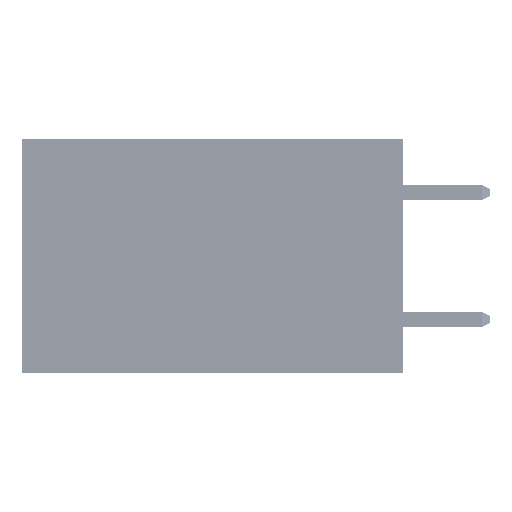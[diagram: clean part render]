
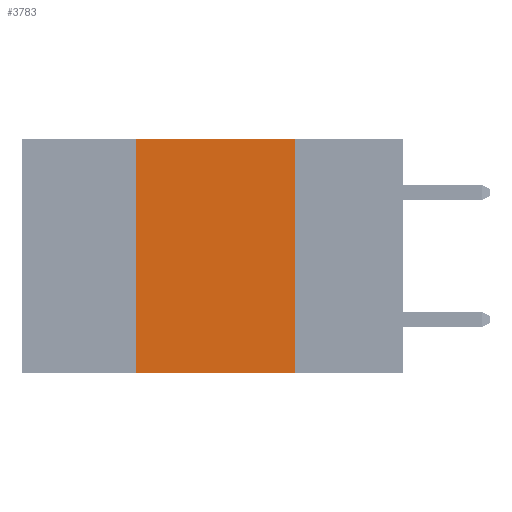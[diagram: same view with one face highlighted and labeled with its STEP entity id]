
A CAD part, left-side view. The second image highlights one B-rep face of the part: STEP entity #3783.
In plain terms, the highlighted planar face has unit normal (-1, 0, 0).
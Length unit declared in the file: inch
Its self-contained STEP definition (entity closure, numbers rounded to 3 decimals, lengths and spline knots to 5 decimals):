
#2106 = LINE ( 'NONE', #50975, #31620 ) ;
#3321 = PLANE ( 'NONE',  #11243 ) ;
#3783 = ADVANCED_FACE ( 'NONE', ( #17628 ), #3321, .F. ) ;
#4459 = EDGE_CURVE ( 'NONE', #30673, #30750, #28475, .T. ) ;
#5529 = EDGE_CURVE ( 'NONE', #30750, #41120, #49091, .T. ) ;
#6815 = DIRECTION ( 'NONE',  ( 0., 0., -1. ) ) ;
#7214 = DIRECTION ( 'NONE',  ( 0., 0., -1. ) ) ;
#10422 = VECTOR ( 'NONE', #35264, 39.37008 ) ;
#11243 = AXIS2_PLACEMENT_3D ( 'NONE', #31397, #50883, #7214 ) ;
#11581 = CARTESIAN_POINT ( 'NONE',  ( 0., 0.6, -0.37 ) ) ;
#11615 = CARTESIAN_POINT ( 'NONE',  ( 0., 0.17, -0.37 ) ) ;
#12536 = CARTESIAN_POINT ( 'NONE',  ( 0., 0.6, 0. ) ) ;
#15383 = EDGE_CURVE ( 'NONE', #51224, #41120, #46801, .T. ) ;
#16213 = ORIENTED_EDGE ( 'NONE', *, *, #47857, .F. ) ;
#16695 = CARTESIAN_POINT ( 'NONE',  ( 0., 0.42, 0. ) ) ;
#17628 = FACE_OUTER_BOUND ( 'NONE', #46523, .T. ) ;
#27296 = DIRECTION ( 'NONE',  ( 0., 0., 1. ) ) ;
#28458 = DIRECTION ( 'NONE',  ( 0., -1., 0. ) ) ;
#28475 = LINE ( 'NONE', #12536, #51683 ) ;
#29568 = ORIENTED_EDGE ( 'NONE', *, *, #15383, .T. ) ;
#30673 = VERTEX_POINT ( 'NONE', #16695 ) ;
#30750 = VERTEX_POINT ( 'NONE', #37182 ) ;
#31397 = CARTESIAN_POINT ( 'NONE',  ( 0., 0.6, 0. ) ) ;
#31620 = VECTOR ( 'NONE', #27296, 39.37008 ) ;
#35136 = ORIENTED_EDGE ( 'NONE', *, *, #4459, .F. ) ;
#35264 = DIRECTION ( 'NONE',  ( 0., -1., 0. ) ) ;
#36014 = ORIENTED_EDGE ( 'NONE', *, *, #5529, .F. ) ;
#37182 = CARTESIAN_POINT ( 'NONE',  ( 0., 0.17, 0. ) ) ;
#38834 = CARTESIAN_POINT ( 'NONE',  ( 0., 0.42, -0.37 ) ) ;
#41120 = VERTEX_POINT ( 'NONE', #11615 ) ;
#42192 = VECTOR ( 'NONE', #6815, 39.37008 ) ;
#46449 = CARTESIAN_POINT ( 'NONE',  ( 0., 0.17, 0. ) ) ;
#46523 = EDGE_LOOP ( 'NONE', ( #36014, #35136, #16213, #29568 ) ) ;
#46801 = LINE ( 'NONE', #11581, #10422 ) ;
#47857 = EDGE_CURVE ( 'NONE', #51224, #30673, #2106, .T. ) ;
#49091 = LINE ( 'NONE', #46449, #42192 ) ;
#50883 = DIRECTION ( 'NONE',  ( 1., 0., 0. ) ) ;
#50975 = CARTESIAN_POINT ( 'NONE',  ( 0., 0.42, 0. ) ) ;
#51224 = VERTEX_POINT ( 'NONE', #38834 ) ;
#51683 = VECTOR ( 'NONE', #28458, 39.37008 ) ;
